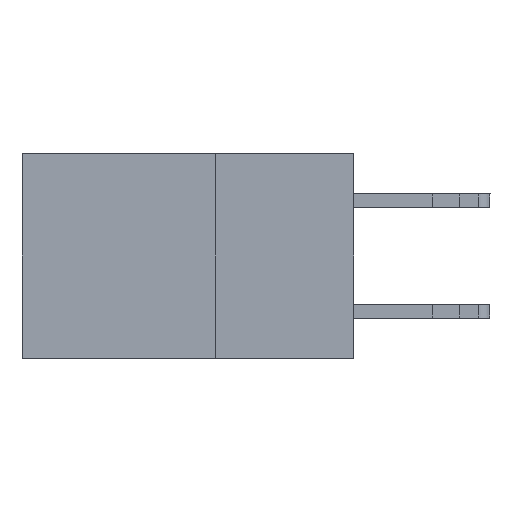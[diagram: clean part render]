
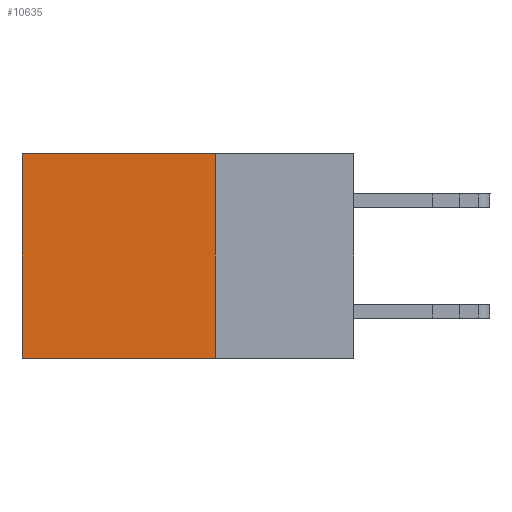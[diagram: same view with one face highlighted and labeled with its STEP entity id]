
A CAD part, left-side view. The second image highlights one B-rep face of the part: STEP entity #10635.
In plain terms, the highlighted planar face has unit normal (-1, 0, 0).
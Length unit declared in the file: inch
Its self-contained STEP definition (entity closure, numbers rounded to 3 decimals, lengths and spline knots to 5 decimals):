
#231 = EDGE_CURVE ( 'NONE', #16066, #5475, #4433, .T. ) ;
#269 = VERTEX_POINT ( 'NONE', #1895 ) ;
#1664 = EDGE_LOOP ( 'NONE', ( #18080, #2353, #17040, #18058 ) ) ;
#1822 = VECTOR ( 'NONE', #7608, 39.37008 ) ;
#1895 = CARTESIAN_POINT ( 'NONE',  ( 0.2875, 0.6, 0. ) ) ;
#2353 = ORIENTED_EDGE ( 'NONE', *, *, #13165, .F. ) ;
#2406 = CARTESIAN_POINT ( 'NONE',  ( 0.2875, 0.25, 0. ) ) ;
#2992 = DIRECTION ( 'NONE',  ( 0., 0., -1. ) ) ;
#4433 = LINE ( 'NONE', #15075, #1822 ) ;
#4646 = CARTESIAN_POINT ( 'NONE',  ( 0.2875, 0.25, -0.37 ) ) ;
#4734 = LINE ( 'NONE', #4646, #11650 ) ;
#5475 = VERTEX_POINT ( 'NONE', #9987 ) ;
#6787 = FACE_OUTER_BOUND ( 'NONE', #1664, .T. ) ;
#7608 = DIRECTION ( 'NONE',  ( 0., 0., -1. ) ) ;
#7623 = DIRECTION ( 'NONE',  ( 0., 1., 0. ) ) ;
#8675 = EDGE_CURVE ( 'NONE', #269, #9871, #16646, .T. ) ;
#9871 = VERTEX_POINT ( 'NONE', #13383 ) ;
#9987 = CARTESIAN_POINT ( 'NONE',  ( 0.2875, 0.25, -0.37 ) ) ;
#10635 = ADVANCED_FACE ( 'NONE', ( #6787 ), #18723, .F. ) ;
#10949 = VECTOR ( 'NONE', #2992, 39.37008 ) ;
#11035 = VECTOR ( 'NONE', #18234, 39.37008 ) ;
#11650 = VECTOR ( 'NONE', #7623, 39.37008 ) ;
#12954 = DIRECTION ( 'NONE',  ( 1., 0., 0. ) ) ;
#13165 = EDGE_CURVE ( 'NONE', #5475, #9871, #4734, .T. ) ;
#13383 = CARTESIAN_POINT ( 'NONE',  ( 0.2875, 0.6, -0.37 ) ) ;
#13521 = AXIS2_PLACEMENT_3D ( 'NONE', #2406, #12954, #18927 ) ;
#13751 = CARTESIAN_POINT ( 'NONE',  ( 0.2875, 0.25, 0. ) ) ;
#14037 = EDGE_CURVE ( 'NONE', #16066, #269, #18616, .T. ) ;
#15075 = CARTESIAN_POINT ( 'NONE',  ( 0.2875, 0.25, 0. ) ) ;
#15520 = CARTESIAN_POINT ( 'NONE',  ( 0.2875, 0.6, 0. ) ) ;
#16066 = VERTEX_POINT ( 'NONE', #19282 ) ;
#16646 = LINE ( 'NONE', #15520, #10949 ) ;
#17040 = ORIENTED_EDGE ( 'NONE', *, *, #231, .F. ) ;
#18058 = ORIENTED_EDGE ( 'NONE', *, *, #14037, .T. ) ;
#18080 = ORIENTED_EDGE ( 'NONE', *, *, #8675, .T. ) ;
#18234 = DIRECTION ( 'NONE',  ( 0., 1., 0. ) ) ;
#18616 = LINE ( 'NONE', #13751, #11035 ) ;
#18723 = PLANE ( 'NONE',  #13521 ) ;
#18927 = DIRECTION ( 'NONE',  ( 0., 0., -1. ) ) ;
#19282 = CARTESIAN_POINT ( 'NONE',  ( 0.2875, 0.25, 0. ) ) ;
